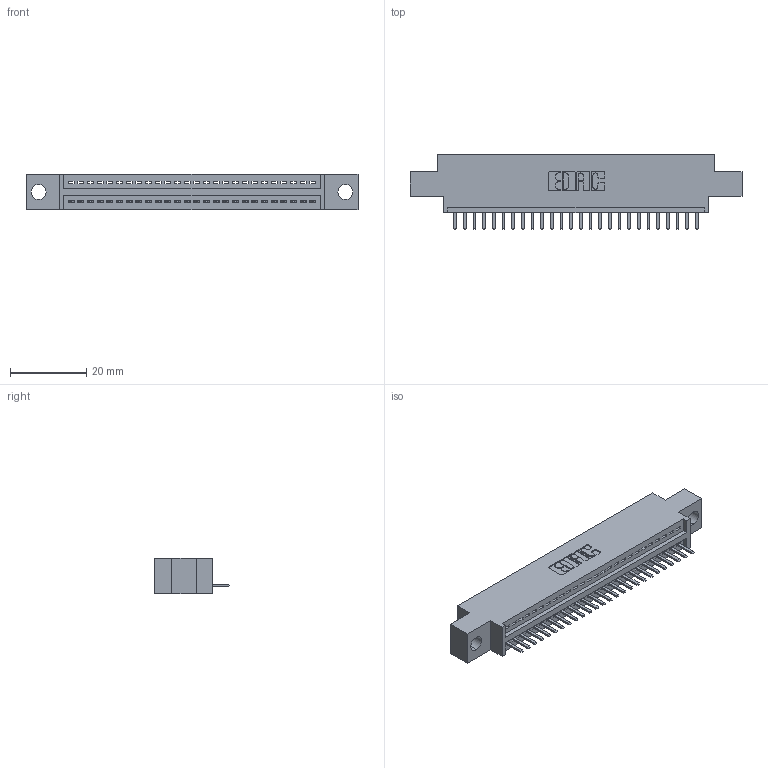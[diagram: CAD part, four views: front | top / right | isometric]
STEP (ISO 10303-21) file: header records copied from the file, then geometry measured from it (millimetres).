
FILE_DESCRIPTION (( 'STEP AP203' ), '1' );
FILE_NAME ('395-026-520-604.STEP', '2018-11-09T15:46:40', ( '' ), ( '' ), 'SwSTEP 2.0', 'SolidWorks 2016', '' );
FILE_SCHEMA (( 'CONFIG_CONTROL_DESIGN' ));
Length unit declared in the file: inch
Products named in the file (3): 345-292-001_345-293-120; 345 Part_0.170 Offset - 0.156 Dia-TH; 395-026-520-604
Assembly tree (27 placements, depth 2):
  395-026-520-604
    345 Part_0.170 Offset - 0.156 Dia-TH
    345-292-001_345-293-120  x26
Bounding box: 87.25 x 19.68 x 9.4 mm (x, y, z)
Volume: 7879.9 mm3; surface area: 9944.9 mm2
Topology: 27 solids, 27 shells, 1742 faces, 5137 edges, 3354 vertices
Faces by surface type: plane 1176, cylinder 566
Entity records: 21971 total; most frequent: CARTESIAN_POINT 3826, ORIENTED_EDGE 3774, DIRECTION 3351, EDGE_CURVE 1887, LINE 1647, VECTOR 1647, VERTEX_POINT 1254, AXIS2_PLACEMENT_3D 852
